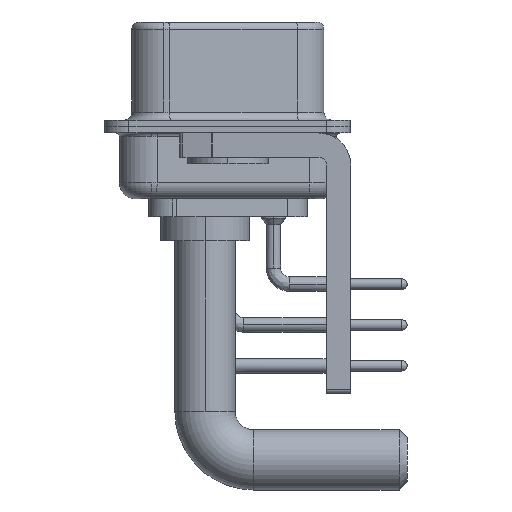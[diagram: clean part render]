
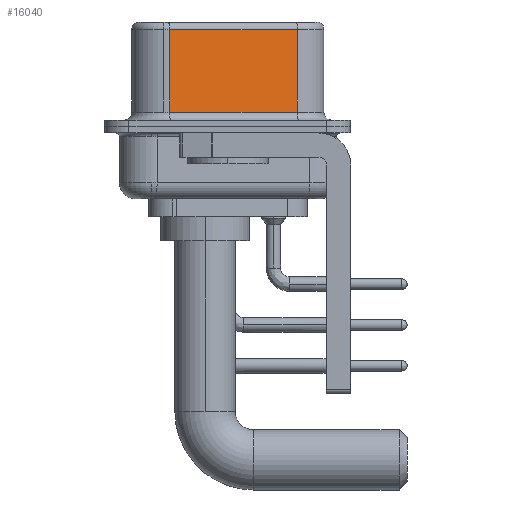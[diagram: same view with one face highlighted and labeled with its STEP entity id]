
A CAD part, left-side view. The second image highlights one B-rep face of the part: STEP entity #16040.
In plain terms, the highlighted planar face has unit normal (-0.985, -0.174, 0).
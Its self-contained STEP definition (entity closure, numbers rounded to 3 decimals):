
#510 = FACE_OUTER_BOUND ( 'NONE', #10855, .T. ) ;
#3941 = LINE ( 'NONE', #11757, #31934 ) ;
#5815 = EDGE_CURVE ( 'NONE', #13019, #27468, #31633, .T. ) ;
#8834 = CARTESIAN_POINT ( 'NONE',  ( 5.132, -4.322, 6.52 ) ) ;
#9099 = DIRECTION ( 'NONE',  ( -0.174, 0.985, 0. ) ) ;
#9991 = ORIENTED_EDGE ( 'NONE', *, *, #17122, .T. ) ;
#10154 = DIRECTION ( 'NONE',  ( 0., 0., -1. ) ) ;
#10203 = CARTESIAN_POINT ( 'NONE',  ( 5.132, -4.322, 6.02 ) ) ;
#10855 = EDGE_LOOP ( 'NONE', ( #17427, #28238, #27239, #9991 ) ) ;
#10947 = DIRECTION ( 'NONE',  ( -0.174, 0.985, 0. ) ) ;
#11533 = AXIS2_PLACEMENT_3D ( 'NONE', #8834, #19282, #10947 ) ;
#11757 = CARTESIAN_POINT ( 'NONE',  ( 5.132, -4.322, 6.02 ) ) ;
#12140 = VECTOR ( 'NONE', #12241, 1000. ) ;
#12241 = DIRECTION ( 'NONE',  ( 0.174, -0.985, 0. ) ) ;
#13019 = VERTEX_POINT ( 'NONE', #29288 ) ;
#15751 = VERTEX_POINT ( 'NONE', #23377 ) ;
#16040 = ADVANCED_FACE ( 'NONE', ( #510 ), #27263, .F. ) ;
#16252 = VERTEX_POINT ( 'NONE', #10203 ) ;
#16395 = VECTOR ( 'NONE', #10154, 1000. ) ;
#17122 = EDGE_CURVE ( 'NONE', #27468, #15751, #17551, .T. ) ;
#17427 = ORIENTED_EDGE ( 'NONE', *, *, #34610, .F. ) ;
#17551 = LINE ( 'NONE', #28361, #12140 ) ;
#17684 = VECTOR ( 'NONE', #26699, 1000. ) ;
#19282 = DIRECTION ( 'NONE',  ( 0.985, 0.174, 0. ) ) ;
#23377 = CARTESIAN_POINT ( 'NONE',  ( 5.132, -4.322, 0.9 ) ) ;
#23983 = LINE ( 'NONE', #26479, #16395 ) ;
#26432 = EDGE_CURVE ( 'NONE', #16252, #13019, #3941, .T. ) ;
#26479 = CARTESIAN_POINT ( 'NONE',  ( 5.132, -4.322, 6.52 ) ) ;
#26699 = DIRECTION ( 'NONE',  ( 0., 0., -1. ) ) ;
#27239 = ORIENTED_EDGE ( 'NONE', *, *, #5815, .T. ) ;
#27263 = PLANE ( 'NONE',  #11533 ) ;
#27468 = VERTEX_POINT ( 'NONE', #31890 ) ;
#28238 = ORIENTED_EDGE ( 'NONE', *, *, #26432, .T. ) ;
#28361 = CARTESIAN_POINT ( 'NONE',  ( 5.132, -4.322, 0.9 ) ) ;
#29288 = CARTESIAN_POINT ( 'NONE',  ( 3.73, 3.628, 6.02 ) ) ;
#31633 = LINE ( 'NONE', #32164, #17684 ) ;
#31890 = CARTESIAN_POINT ( 'NONE',  ( 3.73, 3.628, 0.9 ) ) ;
#31934 = VECTOR ( 'NONE', #9099, 1000. ) ;
#32164 = CARTESIAN_POINT ( 'NONE',  ( 3.73, 3.628, 6.52 ) ) ;
#34610 = EDGE_CURVE ( 'NONE', #16252, #15751, #23983, .T. ) ;
